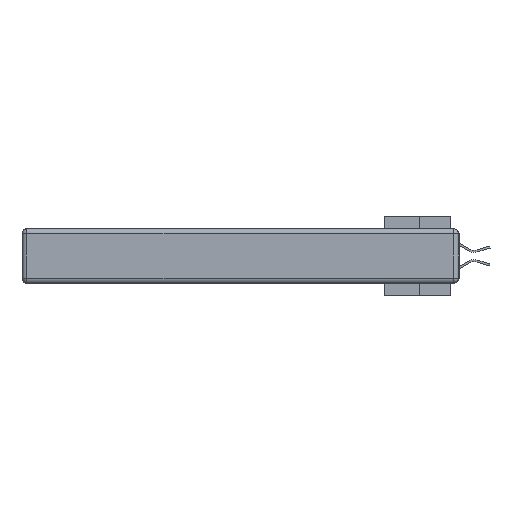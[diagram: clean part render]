
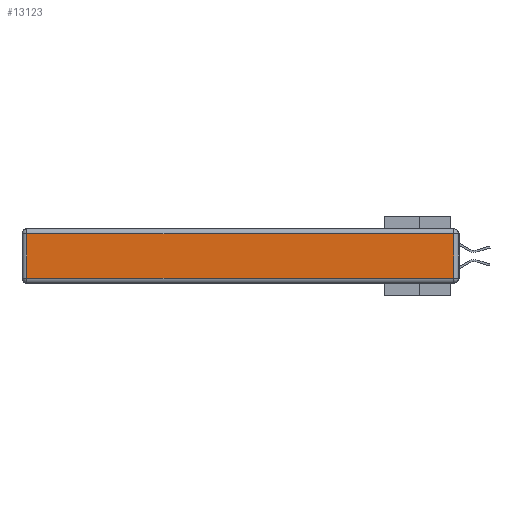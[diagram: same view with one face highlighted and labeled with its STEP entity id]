
A CAD part, left-side view. The second image highlights one B-rep face of the part: STEP entity #13123.
In plain terms, the highlighted planar face has unit normal (-1, 0, 0).
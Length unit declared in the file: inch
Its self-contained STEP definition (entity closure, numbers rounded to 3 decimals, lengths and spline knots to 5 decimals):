
#326 = CARTESIAN_POINT ( 'NONE',  ( 0., 0., -0.343 ) ) ;
#367 = VECTOR ( 'NONE', #15446, 39.37008 ) ;
#961 = LINE ( 'NONE', #23636, #27454 ) ;
#2398 = ORIENTED_EDGE ( 'NONE', *, *, #12865, .T. ) ;
#3859 = CARTESIAN_POINT ( 'NONE',  ( 0., 2.72, -0.03 ) ) ;
#4623 = CARTESIAN_POINT ( 'NONE',  ( 0., 0.03, -0.03 ) ) ;
#4761 = LINE ( 'NONE', #17513, #17457 ) ;
#5479 = DIRECTION ( 'NONE',  ( -1., 0., 0. ) ) ;
#5648 = CARTESIAN_POINT ( 'NONE',  ( 0., 2.75, -0.03 ) ) ;
#6891 = LINE ( 'NONE', #9204, #7640 ) ;
#7640 = VECTOR ( 'NONE', #13728, 39.37008 ) ;
#7968 = EDGE_LOOP ( 'NONE', ( #2398, #15167, #15761, #23792 ) ) ;
#9204 = CARTESIAN_POINT ( 'NONE',  ( 0., 2.72, -0.343 ) ) ;
#9239 = LINE ( 'NONE', #5648, #367 ) ;
#10371 = VERTEX_POINT ( 'NONE', #20275 ) ;
#10452 = EDGE_CURVE ( 'NONE', #12964, #27735, #9239, .T. ) ;
#12322 = CARTESIAN_POINT ( 'NONE',  ( 0., 2.72, -0.313 ) ) ;
#12865 = EDGE_CURVE ( 'NONE', #27469, #10371, #961, .T. ) ;
#12964 = VERTEX_POINT ( 'NONE', #4623 ) ;
#13123 = ADVANCED_FACE ( 'NONE', ( #19025 ), #15301, .T. ) ;
#13650 = EDGE_CURVE ( 'NONE', #10371, #12964, #4761, .T. ) ;
#13728 = DIRECTION ( 'NONE',  ( 0., 0., -1. ) ) ;
#14851 = DIRECTION ( 'NONE',  ( 0., 0., 1. ) ) ;
#15167 = ORIENTED_EDGE ( 'NONE', *, *, #13650, .T. ) ;
#15301 = PLANE ( 'NONE',  #22107 ) ;
#15446 = DIRECTION ( 'NONE',  ( 0., 1., 0. ) ) ;
#15761 = ORIENTED_EDGE ( 'NONE', *, *, #10452, .T. ) ;
#17457 = VECTOR ( 'NONE', #14851, 39.37008 ) ;
#17513 = CARTESIAN_POINT ( 'NONE',  ( 0., 0.03, -0.343 ) ) ;
#17554 = DIRECTION ( 'NONE',  ( 0., 0., 1. ) ) ;
#19025 = FACE_OUTER_BOUND ( 'NONE', #7968, .T. ) ;
#20037 = EDGE_CURVE ( 'NONE', #27735, #27469, #6891, .T. ) ;
#20275 = CARTESIAN_POINT ( 'NONE',  ( 0., 0.03, -0.313 ) ) ;
#21409 = DIRECTION ( 'NONE',  ( 0., -1., 0. ) ) ;
#22107 = AXIS2_PLACEMENT_3D ( 'NONE', #326, #5479, #17554 ) ;
#23636 = CARTESIAN_POINT ( 'NONE',  ( 0., 0., -0.313 ) ) ;
#23792 = ORIENTED_EDGE ( 'NONE', *, *, #20037, .T. ) ;
#27454 = VECTOR ( 'NONE', #21409, 39.37008 ) ;
#27469 = VERTEX_POINT ( 'NONE', #12322 ) ;
#27735 = VERTEX_POINT ( 'NONE', #3859 ) ;
